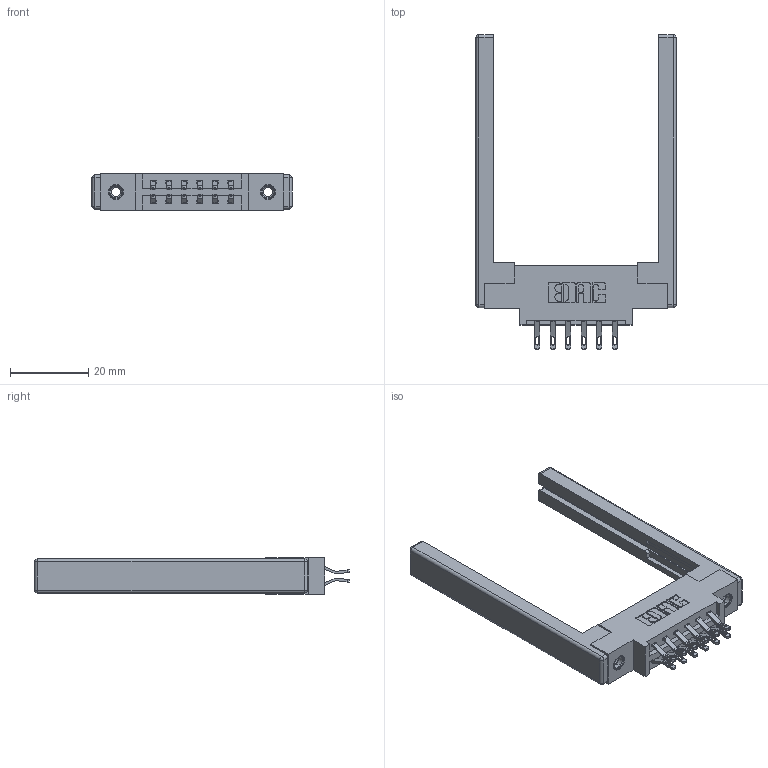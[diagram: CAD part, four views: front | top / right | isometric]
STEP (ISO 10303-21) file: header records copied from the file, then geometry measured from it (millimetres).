
FILE_DESCRIPTION (( 'STEP AP203' ), '1' );
FILE_NAME ('337-012-555-868.STEP', '2019-10-10T16:16:39', ( '' ), ( '' ), 'SwSTEP 2.0', 'SolidWorks 2016', '' );
FILE_SCHEMA (( 'CONFIG_CONTROL_DESIGN' ));
Length unit declared in the file: inch
Products named in the file (5): 307-220-068; 345-292-001_555 Tail; 337 Part_0.170 Offset - 0.156 Dia-TI; 345-250-001_345-250-001-102; 337-012-555-868
Assembly tree (17 placements, depth 2):
  337-012-555-868
    337 Part_0.170 Offset - 0.156 Dia-TI
    345-292-001_555 Tail  x12
    345-250-001_345-250-001-102  x2
    307-220-068  x2
Bounding box: 51.21 x 80.52 x 9.4 mm (x, y, z)
Volume: 9219.4 mm3; surface area: 9389.2 mm2
Topology: 17 solids, 17 shells, 992 faces, 2981 edges, 1966 vertices
Faces by surface type: plane 594, cylinder 374, cone 12, sphere 8, torus 4
Entity records: 12526 total; most frequent: CARTESIAN_POINT 2141, ORIENTED_EDGE 2036, DIRECTION 1928, EDGE_CURVE 1018, LINE 820, VECTOR 820, VERTEX_POINT 670, AXIS2_PLACEMENT_3D 554
